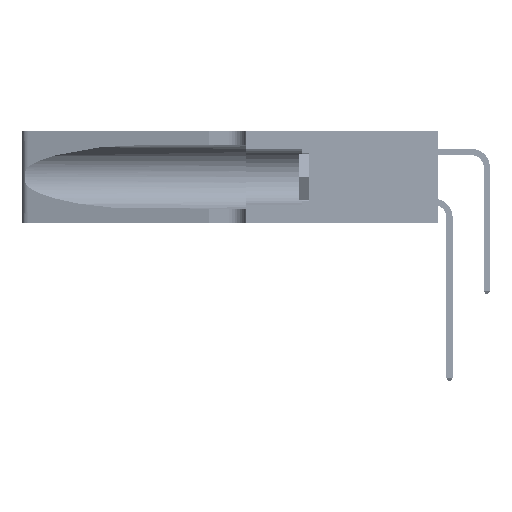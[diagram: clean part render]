
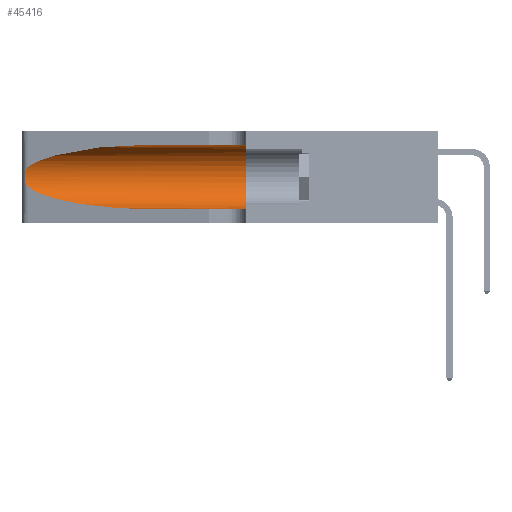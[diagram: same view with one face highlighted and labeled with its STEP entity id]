
A CAD part, left-side view. The second image highlights one B-rep face of the part: STEP entity #45416.
In plain terms, the highlighted cylindrical face has radius 3.308 mm (diameter 6.617 mm), a partial arc.
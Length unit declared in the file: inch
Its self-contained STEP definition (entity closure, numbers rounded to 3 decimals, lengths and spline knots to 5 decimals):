
#891 = CIRCLE ( 'NONE', #13348, 0.13025 ) ;
#2911 = CARTESIAN_POINT ( 'NONE',  ( 0.1305, 1.61858, 0.185 ) ) ;
#3127 = DIRECTION ( 'NONE',  ( 0., 0., 1. ) ) ;
#3238 = CARTESIAN_POINT ( 'NONE',  ( 0.26018, 1.23835, 0.19895 ) ) ;
#7391 = DIRECTION ( 'NONE',  ( 0., -1., 0. ) ) ;
#7554 = EDGE_CURVE ( 'NONE', #17680, #43918, #18835, .T. ) ;
#7736 = CARTESIAN_POINT ( 'NONE',  ( 0.26075, 1.23896, 0.178 ) ) ;
#8066 = VERTEX_POINT ( 'NONE', #53946 ) ;
#10735 = CARTESIAN_POINT ( 'NONE',  ( 0.1305, 0.72297, 0.31525 ) ) ;
#12029 = VECTOR ( 'NONE', #30967, 39.37008 ) ;
#12185 = CARTESIAN_POINT ( 'NONE',  ( 0.25856, 1.23593, 0.16098 ) ) ;
#13348 = AXIS2_PLACEMENT_3D ( 'NONE', #55269, #29369, #3127 ) ;
#14555 = CARTESIAN_POINT ( 'NONE',  ( 0.1305, 0.72297, 0.31525 ) ) ;
#14823 = CARTESIAN_POINT ( 'NONE',  ( 0.18966, 0.96281, 0.05475 ) ) ;
#16412 = CARTESIAN_POINT ( 'NONE',  ( 0.25487, 1.22718, 0.22369 ) ) ;
#16605 = CARTESIAN_POINT ( 'NONE',  ( 0.25639, 1.23186, 0.15144 ) ) ;
#16769 = EDGE_CURVE ( 'NONE', #31529, #8066, #24782, .T. ) ;
#17680 = VERTEX_POINT ( 'NONE', #43062 ) ;
#17981 = ORIENTED_EDGE ( 'NONE', *, *, #16769, .T. ) ;
#18517 = ORIENTED_EDGE ( 'NONE', *, *, #39630, .T. ) ;
#18835 =( BOUNDED_CURVE ( )  B_SPLINE_CURVE ( 3, ( #19207, #32102, #14823, #49459 ),
 .UNSPECIFIED., .F., .F. ) 
 B_SPLINE_CURVE_WITH_KNOTS ( ( 4, 4 ),
 ( 3.44316, 4.71239 ),
 .UNSPECIFIED. ) 
 CURVE ( )  GEOMETRIC_REPRESENTATION_ITEM ( )  RATIONAL_B_SPLINE_CURVE ( ( 1., 0.87, 0.87, 1. ) ) 
 REPRESENTATION_ITEM ( '' )  );
#18930 = CARTESIAN_POINT ( 'NONE',  ( 0.18966, 0.96281, 0.31525 ) ) ;
#19207 = CARTESIAN_POINT ( 'NONE',  ( 0.25487, 1.22718, 0.14631 ) ) ;
#19985 = VERTEX_POINT ( 'NONE', #43657 ) ;
#20614 = B_SPLINE_CURVE_WITH_KNOTS ( 'NONE', 3,
 ( #16412, #20812, #25166, #55372, #29483, #3238, #33837, #7736, #38200, #12185, #42516, #16605, #46897, #20990 ),
 .UNSPECIFIED., .F., .F.,
 ( 4, 2, 2, 2, 2, 2, 4 ),
 ( 0., 0.00027, 0.00053, 0.00107, 0.0016, 0.00187, 0.00214 ),
 .UNSPECIFIED. ) ;
#20812 = CARTESIAN_POINT ( 'NONE',  ( 0.25555, 1.22994, 0.2215 ) ) ;
#20990 = CARTESIAN_POINT ( 'NONE',  ( 0.25487, 1.22718, 0.14631 ) ) ;
#21009 = EDGE_CURVE ( 'NONE', #19985, #31443, #891, .T. ) ;
#21582 = EDGE_LOOP ( 'NONE', ( #17981, #18517, #22854, #23618, #24092, #31561 ) ) ;
#22854 = ORIENTED_EDGE ( 'NONE', *, *, #7554, .T. ) ;
#22993 = CARTESIAN_POINT ( 'NONE',  ( 0.1305, 0.35, 0.05475 ) ) ;
#23334 = CARTESIAN_POINT ( 'NONE',  ( 0.25487, 1.22718, 0.22369 ) ) ;
#23618 = ORIENTED_EDGE ( 'NONE', *, *, #45353, .T. ) ;
#24092 = ORIENTED_EDGE ( 'NONE', *, *, #21009, .F. ) ;
#24227 = CYLINDRICAL_SURFACE ( 'NONE', #32098, 0.13025 ) ;
#24272 = CARTESIAN_POINT ( 'NONE',  ( 0.1305, 1.61858, 0.05475 ) ) ;
#24782 =( BOUNDED_CURVE ( )  B_SPLINE_CURVE ( 3, ( #14555, #18930, #49193, #23334 ),
 .UNSPECIFIED., .F., .F. ) 
 B_SPLINE_CURVE_WITH_KNOTS ( ( 4, 4 ),
 ( 1.5708, 2.84003 ),
 .UNSPECIFIED. ) 
 CURVE ( )  GEOMETRIC_REPRESENTATION_ITEM ( )  RATIONAL_B_SPLINE_CURVE ( ( 1., 0.87, 0.87, 1. ) ) 
 REPRESENTATION_ITEM ( '' )  );
#25166 = CARTESIAN_POINT ( 'NONE',  ( 0.25639, 1.23184, 0.21858 ) ) ;
#26650 = CARTESIAN_POINT ( 'NONE',  ( 0.1305, 1.61858, 0.31525 ) ) ;
#28267 = VECTOR ( 'NONE', #50149, 39.37008 ) ;
#29155 = DIRECTION ( 'NONE',  ( 0., 0., -1. ) ) ;
#29369 = DIRECTION ( 'NONE',  ( 0., 1., 0. ) ) ;
#29483 = CARTESIAN_POINT ( 'NONE',  ( 0.25854, 1.2359, 0.20912 ) ) ;
#30967 = DIRECTION ( 'NONE',  ( 0., -1., 0. ) ) ;
#31443 = VERTEX_POINT ( 'NONE', #22993 ) ;
#31529 = VERTEX_POINT ( 'NONE', #10735 ) ;
#31561 = ORIENTED_EDGE ( 'NONE', *, *, #39873, .F. ) ;
#31573 = CARTESIAN_POINT ( 'NONE',  ( 0.1305, 0.72297, 0.05475 ) ) ;
#32098 = AXIS2_PLACEMENT_3D ( 'NONE', #2911, #7391, #29155 ) ;
#32102 = CARTESIAN_POINT ( 'NONE',  ( 0.2373, 1.15595, 0.08982 ) ) ;
#33837 = CARTESIAN_POINT ( 'NONE',  ( 0.26075, 1.23896, 0.19203 ) ) ;
#38200 = CARTESIAN_POINT ( 'NONE',  ( 0.26017, 1.23833, 0.17102 ) ) ;
#39630 = EDGE_CURVE ( 'NONE', #8066, #17680, #20614, .T. ) ;
#39777 = LINE ( 'NONE', #24272, #28267 ) ;
#39873 = EDGE_CURVE ( 'NONE', #31529, #19985, #46629, .T. ) ;
#42516 = CARTESIAN_POINT ( 'NONE',  ( 0.25789, 1.23486, 0.15765 ) ) ;
#43062 = CARTESIAN_POINT ( 'NONE',  ( 0.25487, 1.22718, 0.14631 ) ) ;
#43657 = CARTESIAN_POINT ( 'NONE',  ( 0.1305, 0.35, 0.31525 ) ) ;
#43918 = VERTEX_POINT ( 'NONE', #31573 ) ;
#45353 = EDGE_CURVE ( 'NONE', #43918, #31443, #39777, .T. ) ;
#45416 = ADVANCED_FACE ( 'NONE', ( #49920 ), #24227, .F. ) ;
#46629 = LINE ( 'NONE', #26650, #12029 ) ;
#46897 = CARTESIAN_POINT ( 'NONE',  ( 0.25555, 1.22993, 0.14849 ) ) ;
#49193 = CARTESIAN_POINT ( 'NONE',  ( 0.2373, 1.15595, 0.28018 ) ) ;
#49459 = CARTESIAN_POINT ( 'NONE',  ( 0.1305, 0.72297, 0.05475 ) ) ;
#49920 = FACE_OUTER_BOUND ( 'NONE', #21582, .T. ) ;
#50149 = DIRECTION ( 'NONE',  ( 0., -1., 0. ) ) ;
#53946 = CARTESIAN_POINT ( 'NONE',  ( 0.25487, 1.22718, 0.22369 ) ) ;
#55269 = CARTESIAN_POINT ( 'NONE',  ( 0.1305, 0.35, 0.185 ) ) ;
#55372 = CARTESIAN_POINT ( 'NONE',  ( 0.25787, 1.23484, 0.2124 ) ) ;
